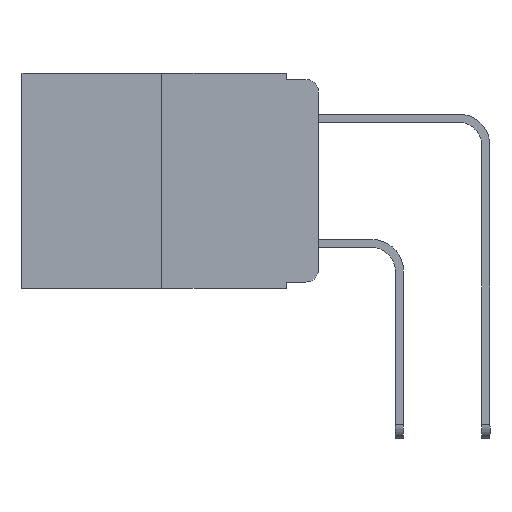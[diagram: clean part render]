
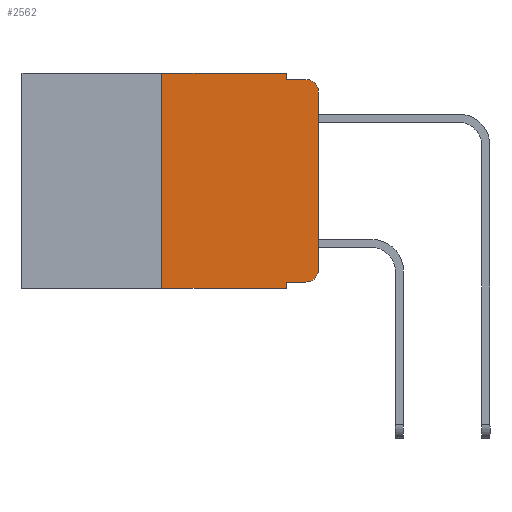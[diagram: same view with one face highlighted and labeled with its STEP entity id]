
A CAD part, left-side view. The second image highlights one B-rep face of the part: STEP entity #2562.
In plain terms, the highlighted planar face has unit normal (-1, 0, 0).
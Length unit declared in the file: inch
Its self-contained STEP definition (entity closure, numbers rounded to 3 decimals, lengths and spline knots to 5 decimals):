
#41 = CARTESIAN_POINT ( 'NONE',  ( 0., 0.051, -0.01 ) ) ;
#88 = VECTOR ( 'NONE', #4937, 39.37008 ) ;
#162 = CARTESIAN_POINT ( 'NONE',  ( 0., 0.25, 0. ) ) ;
#658 = VERTEX_POINT ( 'NONE', #8411 ) ;
#1023 = ORIENTED_EDGE ( 'NONE', *, *, #2822, .F. ) ;
#1271 = CIRCLE ( 'NONE', #8965, 0.02 ) ;
#1586 = VERTEX_POINT ( 'NONE', #15547 ) ;
#1698 = LINE ( 'NONE', #15141, #22126 ) ;
#1893 = CARTESIAN_POINT ( 'NONE',  ( 0., 0.051, -0.01 ) ) ;
#1898 = FACE_OUTER_BOUND ( 'NONE', #20356, .T. ) ;
#2053 = VERTEX_POINT ( 'NONE', #21479 ) ;
#2077 = CARTESIAN_POINT ( 'NONE',  ( 0., 0.25, -0.343 ) ) ;
#2117 = VERTEX_POINT ( 'NONE', #7542 ) ;
#2562 = ADVANCED_FACE ( 'NONE', ( #1898 ), #8898, .F. ) ;
#2822 = EDGE_CURVE ( 'NONE', #7638, #1586, #5094, .T. ) ;
#4188 = CARTESIAN_POINT ( 'NONE',  ( 0., 0.051, 0. ) ) ;
#4353 = CARTESIAN_POINT ( 'NONE',  ( 0., 0.25, 0. ) ) ;
#4759 = DIRECTION ( 'NONE',  ( 0., 0., -1. ) ) ;
#4875 = DIRECTION ( 'NONE',  ( 0., -1., 0. ) ) ;
#4893 = EDGE_CURVE ( 'NONE', #2117, #7099, #19061, .T. ) ;
#4937 = DIRECTION ( 'NONE',  ( 0., 0., 1. ) ) ;
#5094 = LINE ( 'NONE', #41, #18024 ) ;
#5246 = ORIENTED_EDGE ( 'NONE', *, *, #20442, .T. ) ;
#5462 = DIRECTION ( 'NONE',  ( 0., 0., -1. ) ) ;
#5691 = VECTOR ( 'NONE', #4875, 39.37008 ) ;
#5911 = AXIS2_PLACEMENT_3D ( 'NONE', #21227, #14185, #5462 ) ;
#5931 = VERTEX_POINT ( 'NONE', #4353 ) ;
#6008 = LINE ( 'NONE', #4188, #18618 ) ;
#6801 = EDGE_CURVE ( 'NONE', #19769, #2053, #6008, .T. ) ;
#6867 = ORIENTED_EDGE ( 'NONE', *, *, #4893, .T. ) ;
#7066 = DIRECTION ( 'NONE',  ( -1., 0., 0. ) ) ;
#7099 = VERTEX_POINT ( 'NONE', #11597 ) ;
#7161 = DIRECTION ( 'NONE',  ( 0., 0., 1. ) ) ;
#7498 = CIRCLE ( 'NONE', #22584, 0.02 ) ;
#7542 = CARTESIAN_POINT ( 'NONE',  ( 0., 0., -0.313 ) ) ;
#7638 = VERTEX_POINT ( 'NONE', #1893 ) ;
#8411 = CARTESIAN_POINT ( 'NONE',  ( 0., 0.051, 0. ) ) ;
#8898 = PLANE ( 'NONE',  #5911 ) ;
#8965 = AXIS2_PLACEMENT_3D ( 'NONE', #20297, #9700, #17191 ) ;
#9010 = DIRECTION ( 'NONE',  ( 0., -1., 0. ) ) ;
#9074 = EDGE_CURVE ( 'NONE', #5931, #658, #1698, .T. ) ;
#9588 = ORIENTED_EDGE ( 'NONE', *, *, #20526, .T. ) ;
#9700 = DIRECTION ( 'NONE',  ( -1., 0., 0. ) ) ;
#10383 = ORIENTED_EDGE ( 'NONE', *, *, #22098, .F. ) ;
#10628 = CARTESIAN_POINT ( 'NONE',  ( 0., 0.02, -0.333 ) ) ;
#11146 = ORIENTED_EDGE ( 'NONE', *, *, #15385, .F. ) ;
#11597 = CARTESIAN_POINT ( 'NONE',  ( 0., 0., -0.03 ) ) ;
#11676 = ORIENTED_EDGE ( 'NONE', *, *, #18912, .T. ) ;
#11853 = LINE ( 'NONE', #13694, #19487 ) ;
#13466 = DIRECTION ( 'NONE',  ( 0., 0., -1. ) ) ;
#13591 = LINE ( 'NONE', #20624, #5691 ) ;
#13694 = CARTESIAN_POINT ( 'NONE',  ( 0., 0.051, 0. ) ) ;
#14185 = DIRECTION ( 'NONE',  ( 1., 0., 0. ) ) ;
#14897 = VECTOR ( 'NONE', #7161, 39.37008 ) ;
#15141 = CARTESIAN_POINT ( 'NONE',  ( 0., 0.473, 0. ) ) ;
#15268 = CARTESIAN_POINT ( 'NONE',  ( 0., 0., 0. ) ) ;
#15385 = EDGE_CURVE ( 'NONE', #658, #7638, #11853, .T. ) ;
#15434 = ORIENTED_EDGE ( 'NONE', *, *, #19531, .T. ) ;
#15547 = CARTESIAN_POINT ( 'NONE',  ( 0., 0.02, -0.01 ) ) ;
#15799 = CARTESIAN_POINT ( 'NONE',  ( 0., 0.473, -0.343 ) ) ;
#16018 = CARTESIAN_POINT ( 'NONE',  ( 0., 0.02, -0.03 ) ) ;
#17069 = VECTOR ( 'NONE', #9010, 39.37008 ) ;
#17191 = DIRECTION ( 'NONE',  ( 0., 0., -1. ) ) ;
#17282 = DIRECTION ( 'NONE',  ( 0., -1., 0. ) ) ;
#17691 = VERTEX_POINT ( 'NONE', #10628 ) ;
#18024 = VECTOR ( 'NONE', #17282, 39.37008 ) ;
#18618 = VECTOR ( 'NONE', #13466, 39.37008 ) ;
#18636 = ORIENTED_EDGE ( 'NONE', *, *, #9074, .F. ) ;
#18912 = EDGE_CURVE ( 'NONE', #17691, #2117, #1271, .T. ) ;
#19061 = LINE ( 'NONE', #15268, #88 ) ;
#19487 = VECTOR ( 'NONE', #4759, 39.37008 ) ;
#19531 = EDGE_CURVE ( 'NONE', #19769, #17691, #13591, .T. ) ;
#19769 = VERTEX_POINT ( 'NONE', #21644 ) ;
#20081 = LINE ( 'NONE', #162, #14897 ) ;
#20247 = ORIENTED_EDGE ( 'NONE', *, *, #6801, .F. ) ;
#20297 = CARTESIAN_POINT ( 'NONE',  ( 0., 0.02, -0.313 ) ) ;
#20356 = EDGE_LOOP ( 'NONE', ( #6867, #5246, #1023, #11146, #18636, #10383, #9588, #20247, #15434, #11676 ) ) ;
#20442 = EDGE_CURVE ( 'NONE', #7099, #1586, #7498, .T. ) ;
#20526 = EDGE_CURVE ( 'NONE', #21411, #2053, #21265, .T. ) ;
#20624 = CARTESIAN_POINT ( 'NONE',  ( 0., 0.051, -0.333 ) ) ;
#20885 = DIRECTION ( 'NONE',  ( 0., 0., -1. ) ) ;
#21227 = CARTESIAN_POINT ( 'NONE',  ( 0., 0.473, 0. ) ) ;
#21265 = LINE ( 'NONE', #15799, #17069 ) ;
#21411 = VERTEX_POINT ( 'NONE', #2077 ) ;
#21479 = CARTESIAN_POINT ( 'NONE',  ( 0., 0.051, -0.343 ) ) ;
#21644 = CARTESIAN_POINT ( 'NONE',  ( 0., 0.051, -0.333 ) ) ;
#22098 = EDGE_CURVE ( 'NONE', #21411, #5931, #20081, .T. ) ;
#22126 = VECTOR ( 'NONE', #22199, 39.37008 ) ;
#22199 = DIRECTION ( 'NONE',  ( 0., -1., 0. ) ) ;
#22584 = AXIS2_PLACEMENT_3D ( 'NONE', #16018, #7066, #20885 ) ;
